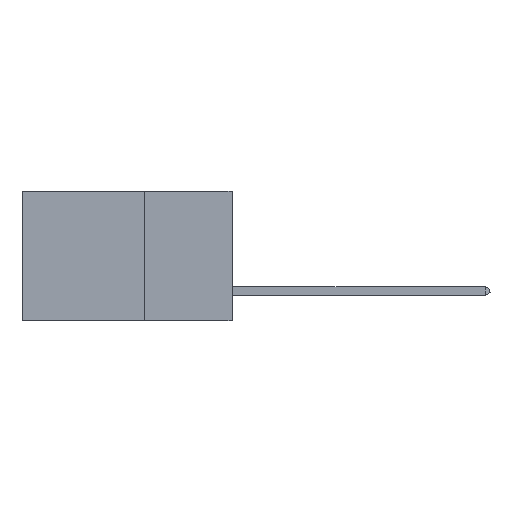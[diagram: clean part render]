
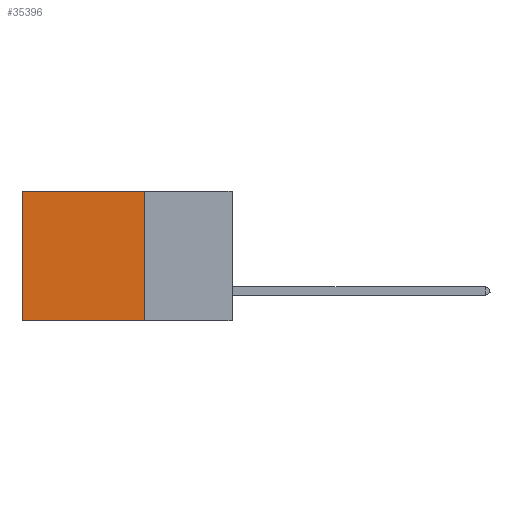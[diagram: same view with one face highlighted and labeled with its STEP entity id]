
A CAD part, left-side view. The second image highlights one B-rep face of the part: STEP entity #35396.
In plain terms, the highlighted planar face has unit normal (-1, 0, 0).
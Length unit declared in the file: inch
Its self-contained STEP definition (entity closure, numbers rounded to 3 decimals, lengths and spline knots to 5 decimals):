
#1197 = LINE ( 'NONE', #13037, #41412 ) ;
#1949 = CARTESIAN_POINT ( 'NONE',  ( 0.2875, 0.6, 0. ) ) ;
#5443 = VERTEX_POINT ( 'NONE', #23945 ) ;
#6471 = LINE ( 'NONE', #1949, #8108 ) ;
#8108 = VECTOR ( 'NONE', #41068, 39.37008 ) ;
#12977 = EDGE_CURVE ( 'NONE', #16419, #17517, #6471, .T. ) ;
#13037 = CARTESIAN_POINT ( 'NONE',  ( 0.2875, 0.25, -0.37 ) ) ;
#13501 = EDGE_CURVE ( 'NONE', #5443, #16419, #27304, .T. ) ;
#16419 = VERTEX_POINT ( 'NONE', #19075 ) ;
#17517 = VERTEX_POINT ( 'NONE', #35289 ) ;
#18030 = ORIENTED_EDGE ( 'NONE', *, *, #13501, .T. ) ;
#18461 = CARTESIAN_POINT ( 'NONE',  ( 0.2875, 0.25, 0. ) ) ;
#19075 = CARTESIAN_POINT ( 'NONE',  ( 0.2875, 0.6, 0. ) ) ;
#19554 = VERTEX_POINT ( 'NONE', #24499 ) ;
#22519 = PLANE ( 'NONE',  #41591 ) ;
#22939 = EDGE_CURVE ( 'NONE', #5443, #19554, #24946, .T. ) ;
#23945 = CARTESIAN_POINT ( 'NONE',  ( 0.2875, 0.25, 0. ) ) ;
#24318 = ORIENTED_EDGE ( 'NONE', *, *, #22939, .F. ) ;
#24499 = CARTESIAN_POINT ( 'NONE',  ( 0.2875, 0.25, -0.37 ) ) ;
#24946 = LINE ( 'NONE', #36179, #30379 ) ;
#27304 = LINE ( 'NONE', #18461, #42668 ) ;
#27454 = EDGE_CURVE ( 'NONE', #19554, #17517, #1197, .T. ) ;
#29408 = DIRECTION ( 'NONE',  ( 1., 0., 0. ) ) ;
#29709 = DIRECTION ( 'NONE',  ( 0., 0., -1. ) ) ;
#30379 = VECTOR ( 'NONE', #32910, 39.37008 ) ;
#30511 = ORIENTED_EDGE ( 'NONE', *, *, #27454, .F. ) ;
#32910 = DIRECTION ( 'NONE',  ( 0., 0., -1. ) ) ;
#34339 = FACE_OUTER_BOUND ( 'NONE', #37473, .T. ) ;
#35289 = CARTESIAN_POINT ( 'NONE',  ( 0.2875, 0.6, -0.37 ) ) ;
#35396 = ADVANCED_FACE ( 'NONE', ( #34339 ), #22519, .F. ) ;
#36179 = CARTESIAN_POINT ( 'NONE',  ( 0.2875, 0.25, 0. ) ) ;
#37473 = EDGE_LOOP ( 'NONE', ( #39345, #30511, #24318, #18030 ) ) ;
#37677 = DIRECTION ( 'NONE',  ( 0., 1., 0. ) ) ;
#39345 = ORIENTED_EDGE ( 'NONE', *, *, #12977, .T. ) ;
#39949 = CARTESIAN_POINT ( 'NONE',  ( 0.2875, 0.25, 0. ) ) ;
#41068 = DIRECTION ( 'NONE',  ( 0., 0., -1. ) ) ;
#41412 = VECTOR ( 'NONE', #37677, 39.37008 ) ;
#41591 = AXIS2_PLACEMENT_3D ( 'NONE', #39949, #29408, #29709 ) ;
#42668 = VECTOR ( 'NONE', #43097, 39.37008 ) ;
#43097 = DIRECTION ( 'NONE',  ( 0., 1., 0. ) ) ;
